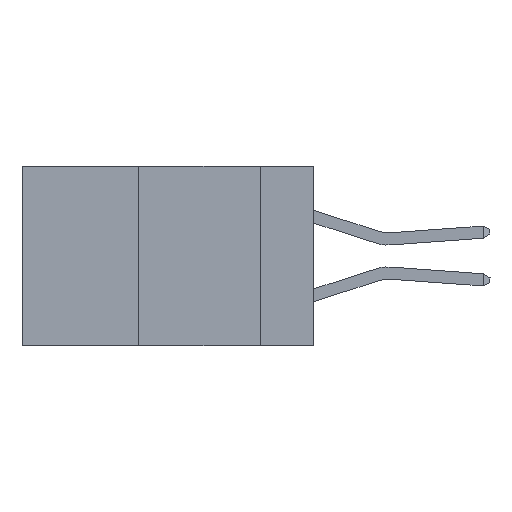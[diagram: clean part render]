
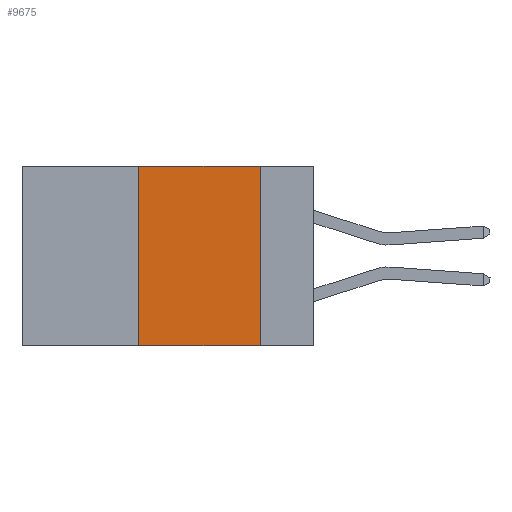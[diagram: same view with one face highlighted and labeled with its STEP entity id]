
A CAD part, left-side view. The second image highlights one B-rep face of the part: STEP entity #9675.
In plain terms, the highlighted planar face has unit normal (-1, 0, 0).
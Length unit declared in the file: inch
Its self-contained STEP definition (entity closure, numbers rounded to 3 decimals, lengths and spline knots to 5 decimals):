
#81 = DIRECTION ( 'NONE',  ( 0., -1., 0. ) ) ;
#550 = ORIENTED_EDGE ( 'NONE', *, *, #5298, .T. ) ;
#1172 = EDGE_CURVE ( 'NONE', #10960, #3944, #12244, .T. ) ;
#1272 = FACE_OUTER_BOUND ( 'NONE', #13562, .T. ) ;
#1560 = DIRECTION ( 'NONE',  ( 0., 0., 1. ) ) ;
#1683 = CARTESIAN_POINT ( 'NONE',  ( 0., 0.36, 0. ) ) ;
#2256 = LINE ( 'NONE', #6002, #10965 ) ;
#2467 = PLANE ( 'NONE',  #4649 ) ;
#2519 = DIRECTION ( 'NONE',  ( 1., 0., 0. ) ) ;
#2737 = CARTESIAN_POINT ( 'NONE',  ( 0., 0.6, 0. ) ) ;
#3944 = VERTEX_POINT ( 'NONE', #7156 ) ;
#4634 = VECTOR ( 'NONE', #9342, 39.37008 ) ;
#4649 = AXIS2_PLACEMENT_3D ( 'NONE', #9393, #2519, #10492 ) ;
#5298 = EDGE_CURVE ( 'NONE', #6059, #6380, #2256, .T. ) ;
#5680 = DIRECTION ( 'NONE',  ( 0., -1., 0. ) ) ;
#6002 = CARTESIAN_POINT ( 'NONE',  ( 0., 0.6, -0.37 ) ) ;
#6032 = ORIENTED_EDGE ( 'NONE', *, *, #1172, .F. ) ;
#6059 = VERTEX_POINT ( 'NONE', #12707 ) ;
#6287 = VECTOR ( 'NONE', #1560, 39.37008 ) ;
#6380 = VERTEX_POINT ( 'NONE', #8150 ) ;
#6895 = EDGE_CURVE ( 'NONE', #6059, #10960, #9336, .T. ) ;
#7156 = CARTESIAN_POINT ( 'NONE',  ( 0., 0.11, 0. ) ) ;
#8150 = CARTESIAN_POINT ( 'NONE',  ( 0., 0.11, -0.37 ) ) ;
#8258 = CARTESIAN_POINT ( 'NONE',  ( 0., 0.11, 0. ) ) ;
#9115 = VECTOR ( 'NONE', #81, 39.37008 ) ;
#9336 = LINE ( 'NONE', #1683, #6287 ) ;
#9342 = DIRECTION ( 'NONE',  ( 0., 0., -1. ) ) ;
#9393 = CARTESIAN_POINT ( 'NONE',  ( 0., 0.6, 0. ) ) ;
#9614 = EDGE_CURVE ( 'NONE', #3944, #6380, #13183, .T. ) ;
#9675 = ADVANCED_FACE ( 'NONE', ( #1272 ), #2467, .F. ) ;
#10492 = DIRECTION ( 'NONE',  ( 0., 0., -1. ) ) ;
#10960 = VERTEX_POINT ( 'NONE', #11843 ) ;
#10965 = VECTOR ( 'NONE', #5680, 39.37008 ) ;
#11652 = ORIENTED_EDGE ( 'NONE', *, *, #9614, .F. ) ;
#11843 = CARTESIAN_POINT ( 'NONE',  ( 0., 0.36, 0. ) ) ;
#11950 = ORIENTED_EDGE ( 'NONE', *, *, #6895, .F. ) ;
#12244 = LINE ( 'NONE', #2737, #9115 ) ;
#12707 = CARTESIAN_POINT ( 'NONE',  ( 0., 0.36, -0.37 ) ) ;
#13183 = LINE ( 'NONE', #8258, #4634 ) ;
#13562 = EDGE_LOOP ( 'NONE', ( #11652, #6032, #11950, #550 ) ) ;
